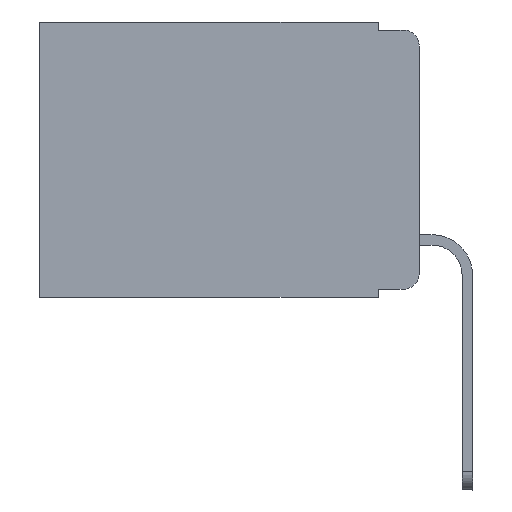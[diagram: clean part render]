
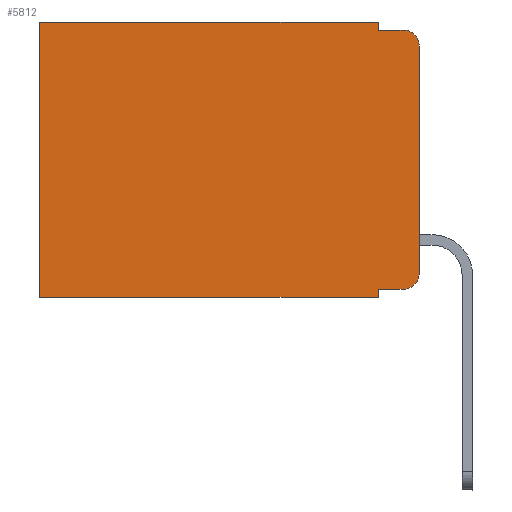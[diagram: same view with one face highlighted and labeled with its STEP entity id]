
A CAD part, left-side view. The second image highlights one B-rep face of the part: STEP entity #5812.
In plain terms, the highlighted planar face has unit normal (-1, 0, 0).
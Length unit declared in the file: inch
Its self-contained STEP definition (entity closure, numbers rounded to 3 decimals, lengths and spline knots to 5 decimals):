
#64 = ORIENTED_EDGE ( 'NONE', *, *, #8074, .F. ) ;
#223 = VERTEX_POINT ( 'NONE', #9506 ) ;
#720 = AXIS2_PLACEMENT_3D ( 'NONE', #8005, #1905, #8251 ) ;
#841 = ORIENTED_EDGE ( 'NONE', *, *, #7856, .F. ) ;
#1080 = CARTESIAN_POINT ( 'NONE',  ( 0.298, 0.02, -0.313 ) ) ;
#1097 = CARTESIAN_POINT ( 'NONE',  ( 0.298, 0.473, 0. ) ) ;
#1746 = LINE ( 'NONE', #13990, #15522 ) ;
#1895 = EDGE_CURVE ( 'NONE', #2884, #12541, #7228, .T. ) ;
#1905 = DIRECTION ( 'NONE',  ( -1., 0., 0. ) ) ;
#1920 = DIRECTION ( 'NONE',  ( 0., 0., -1. ) ) ;
#2108 = DIRECTION ( 'NONE',  ( 0., -1., 0. ) ) ;
#2155 = EDGE_CURVE ( 'NONE', #12168, #12541, #12361, .T. ) ;
#2170 = LINE ( 'NONE', #5739, #8077 ) ;
#2233 = VECTOR ( 'NONE', #2108, 39.37008 ) ;
#2273 = DIRECTION ( 'NONE',  ( 0., 0., -1. ) ) ;
#2531 = LINE ( 'NONE', #14842, #10419 ) ;
#2884 = VERTEX_POINT ( 'NONE', #12707 ) ;
#3249 = DIRECTION ( 'NONE',  ( 1., 0., 0. ) ) ;
#3432 = CARTESIAN_POINT ( 'NONE',  ( 0.298, 0.473, 0. ) ) ;
#3675 = VERTEX_POINT ( 'NONE', #1097 ) ;
#3903 = DIRECTION ( 'NONE',  ( 0., 1., 0. ) ) ;
#4238 = EDGE_CURVE ( 'NONE', #3675, #5672, #15726, .T. ) ;
#4344 = ORIENTED_EDGE ( 'NONE', *, *, #14102, .T. ) ;
#4618 = DIRECTION ( 'NONE',  ( 0., 1., 0. ) ) ;
#4645 = VERTEX_POINT ( 'NONE', #8772 ) ;
#4676 = VECTOR ( 'NONE', #4942, 39.37008 ) ;
#4714 = CARTESIAN_POINT ( 'NONE',  ( 0.298, 0., 0. ) ) ;
#4942 = DIRECTION ( 'NONE',  ( 0., 0., -1. ) ) ;
#5021 = LINE ( 'NONE', #9960, #4676 ) ;
#5307 = CARTESIAN_POINT ( 'NONE',  ( 0.298, 0., -0.03 ) ) ;
#5332 = EDGE_LOOP ( 'NONE', ( #64, #11431, #13410, #841, #8345, #11687, #5378, #10155, #14916, #4344 ) ) ;
#5378 = ORIENTED_EDGE ( 'NONE', *, *, #9336, .F. ) ;
#5672 = VERTEX_POINT ( 'NONE', #12873 ) ;
#5739 = CARTESIAN_POINT ( 'NONE',  ( 0.298, 0., 0. ) ) ;
#5812 = ADVANCED_FACE ( 'NONE', ( #15558 ), #14660, .F. ) ;
#5900 = VERTEX_POINT ( 'NONE', #9662 ) ;
#5934 = EDGE_CURVE ( 'NONE', #223, #11973, #5021, .T. ) ;
#7153 = CARTESIAN_POINT ( 'NONE',  ( 0.298, 0.051, -0.333 ) ) ;
#7178 = DIRECTION ( 'NONE',  ( 0., 0., -1. ) ) ;
#7228 = LINE ( 'NONE', #10774, #2233 ) ;
#7856 = EDGE_CURVE ( 'NONE', #14636, #2884, #1746, .T. ) ;
#8005 = CARTESIAN_POINT ( 'NONE',  ( 0.298, 0.02, -0.03 ) ) ;
#8074 = EDGE_CURVE ( 'NONE', #12168, #4645, #2170, .T. ) ;
#8077 = VECTOR ( 'NONE', #11600, 39.37008 ) ;
#8251 = DIRECTION ( 'NONE',  ( 0., 0., -1. ) ) ;
#8345 = ORIENTED_EDGE ( 'NONE', *, *, #13165, .T. ) ;
#8535 = LINE ( 'NONE', #15700, #13703 ) ;
#8772 = CARTESIAN_POINT ( 'NONE',  ( 0.298, 0., -0.313 ) ) ;
#8978 = CARTESIAN_POINT ( 'NONE',  ( 0.298, 0.02, -0.01 ) ) ;
#9336 = EDGE_CURVE ( 'NONE', #11973, #5672, #2531, .T. ) ;
#9414 = DIRECTION ( 'NONE',  ( 0., -1., 0. ) ) ;
#9506 = CARTESIAN_POINT ( 'NONE',  ( 0.298, 0.051, -0.333 ) ) ;
#9540 = VECTOR ( 'NONE', #9414, 39.37008 ) ;
#9662 = CARTESIAN_POINT ( 'NONE',  ( 0.298, 0.02, -0.333 ) ) ;
#9699 = CARTESIAN_POINT ( 'NONE',  ( 0.298, 0.051, -0.343 ) ) ;
#9960 = CARTESIAN_POINT ( 'NONE',  ( 0.298, 0.051, 0. ) ) ;
#10155 = ORIENTED_EDGE ( 'NONE', *, *, #5934, .F. ) ;
#10419 = VECTOR ( 'NONE', #3903, 39.37008 ) ;
#10774 = CARTESIAN_POINT ( 'NONE',  ( 0.298, 0.051, -0.01 ) ) ;
#11431 = ORIENTED_EDGE ( 'NONE', *, *, #2155, .T. ) ;
#11457 = EDGE_CURVE ( 'NONE', #223, #5900, #12132, .T. ) ;
#11600 = DIRECTION ( 'NONE',  ( 0., 0., -1. ) ) ;
#11687 = ORIENTED_EDGE ( 'NONE', *, *, #4238, .T. ) ;
#11973 = VERTEX_POINT ( 'NONE', #9699 ) ;
#12132 = LINE ( 'NONE', #7153, #9540 ) ;
#12168 = VERTEX_POINT ( 'NONE', #5307 ) ;
#12361 = CIRCLE ( 'NONE', #720, 0.02 ) ;
#12541 = VERTEX_POINT ( 'NONE', #8978 ) ;
#12707 = CARTESIAN_POINT ( 'NONE',  ( 0.298, 0.051, -0.01 ) ) ;
#12789 = CARTESIAN_POINT ( 'NONE',  ( 0.298, 0.051, 0. ) ) ;
#12873 = CARTESIAN_POINT ( 'NONE',  ( 0.298, 0.473, -0.343 ) ) ;
#13165 = EDGE_CURVE ( 'NONE', #14636, #3675, #8535, .T. ) ;
#13410 = ORIENTED_EDGE ( 'NONE', *, *, #1895, .F. ) ;
#13703 = VECTOR ( 'NONE', #4618, 39.37008 ) ;
#13990 = CARTESIAN_POINT ( 'NONE',  ( 0.298, 0.051, 0. ) ) ;
#14102 = EDGE_CURVE ( 'NONE', #5900, #4645, #14978, .T. ) ;
#14636 = VERTEX_POINT ( 'NONE', #12789 ) ;
#14660 = PLANE ( 'NONE',  #15769 ) ;
#14687 = DIRECTION ( 'NONE',  ( 0., 0., -1. ) ) ;
#14773 = DIRECTION ( 'NONE',  ( -1., 0., 0. ) ) ;
#14842 = CARTESIAN_POINT ( 'NONE',  ( 0.298, 0., -0.343 ) ) ;
#14916 = ORIENTED_EDGE ( 'NONE', *, *, #11457, .T. ) ;
#14978 = CIRCLE ( 'NONE', #16010, 0.02 ) ;
#15022 = VECTOR ( 'NONE', #7178, 39.37008 ) ;
#15522 = VECTOR ( 'NONE', #1920, 39.37008 ) ;
#15558 = FACE_OUTER_BOUND ( 'NONE', #5332, .T. ) ;
#15700 = CARTESIAN_POINT ( 'NONE',  ( 0.298, 0., 0. ) ) ;
#15726 = LINE ( 'NONE', #3432, #15022 ) ;
#15769 = AXIS2_PLACEMENT_3D ( 'NONE', #4714, #3249, #2273 ) ;
#16010 = AXIS2_PLACEMENT_3D ( 'NONE', #1080, #14773, #14687 ) ;
